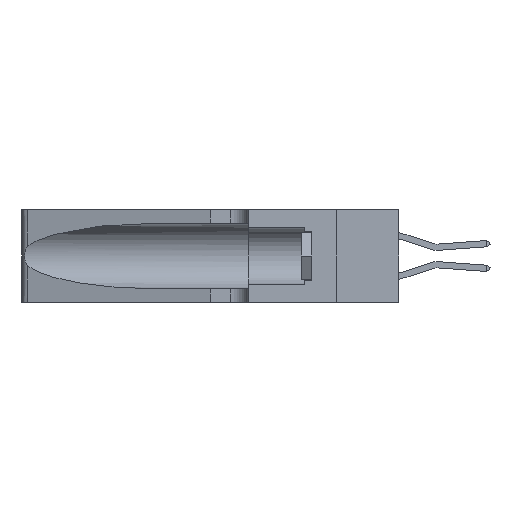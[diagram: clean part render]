
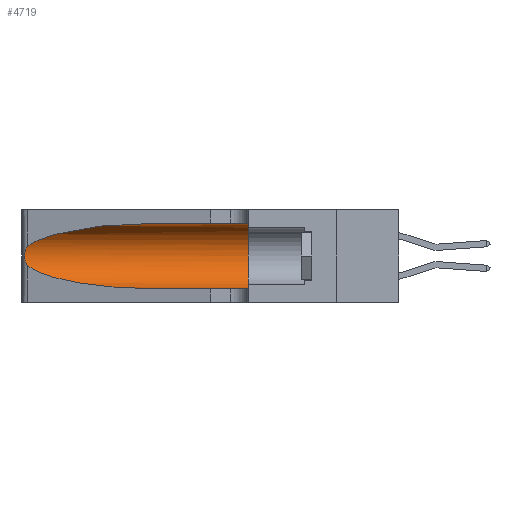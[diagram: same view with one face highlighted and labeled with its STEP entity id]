
A CAD part, left-side view. The second image highlights one B-rep face of the part: STEP entity #4719.
In plain terms, the highlighted cylindrical face has radius 3.308 mm (diameter 6.617 mm), a partial arc.
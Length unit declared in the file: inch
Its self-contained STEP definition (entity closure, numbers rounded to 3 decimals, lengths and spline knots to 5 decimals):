
#1466 = CARTESIAN_POINT ( 'NONE',  ( 0.18966, 0.96281, 0.05475 ) ) ;
#1653 = AXIS2_PLACEMENT_3D ( 'NONE', #7147, #27205, #10057 ) ;
#1807 = CARTESIAN_POINT ( 'NONE',  ( 0.25789, 1.23486, 0.15765 ) ) ;
#2402 = FACE_OUTER_BOUND ( 'NONE', #33620, .T. ) ;
#3666 = VERTEX_POINT ( 'NONE', #22885 ) ;
#3780 = EDGE_CURVE ( 'NONE', #10870, #3666, #19137, .T. ) ;
#3822 = CARTESIAN_POINT ( 'NONE',  ( 0.1305, 0.72297, 0.31525 ) ) ;
#4201 = CARTESIAN_POINT ( 'NONE',  ( 0.1305, 0.72297, 0.05475 ) ) ;
#4461 = DIRECTION ( 'NONE',  ( 0., -1., 0. ) ) ;
#4567 = CARTESIAN_POINT ( 'NONE',  ( 0.25487, 1.22718, 0.22369 ) ) ;
#4694 = CARTESIAN_POINT ( 'NONE',  ( 0.25555, 1.22993, 0.14849 ) ) ;
#4719 = ADVANCED_FACE ( 'NONE', ( #2402 ), #30220, .F. ) ;
#6784 = ORIENTED_EDGE ( 'NONE', *, *, #3780, .F. ) ;
#6940 =( BOUNDED_CURVE ( )  B_SPLINE_CURVE ( 3, ( #23970, #26809, #29705, #12562 ),
 .UNSPECIFIED., .F., .T. ) 
 B_SPLINE_CURVE_WITH_KNOTS ( ( 4, 4 ),
 ( 1.5708, 2.84003 ),
 .UNSPECIFIED. ) 
 CURVE ( )  GEOMETRIC_REPRESENTATION_ITEM ( )  RATIONAL_B_SPLINE_CURVE ( ( 1., 0.87, 0.87, 1. ) ) 
 REPRESENTATION_ITEM ( '' )  );
#7147 = CARTESIAN_POINT ( 'NONE',  ( 0.1305, 0.35, 0.185 ) ) ;
#7508 = CIRCLE ( 'NONE', #1653, 0.13025 ) ;
#7810 = DIRECTION ( 'NONE',  ( 0., -1., 0. ) ) ;
#8117 = ORIENTED_EDGE ( 'NONE', *, *, #17282, .T. ) ;
#9038 = VERTEX_POINT ( 'NONE', #9296 ) ;
#9296 = CARTESIAN_POINT ( 'NONE',  ( 0.25487, 1.22718, 0.22369 ) ) ;
#9963 = CARTESIAN_POINT ( 'NONE',  ( 0.1305, 0.35, 0.05475 ) ) ;
#10057 = DIRECTION ( 'NONE',  ( 0., 0., 1. ) ) ;
#10265 = DIRECTION ( 'NONE',  ( 0., 0., -1. ) ) ;
#10368 = CARTESIAN_POINT ( 'NONE',  ( 0.25787, 1.23484, 0.2124 ) ) ;
#10589 = VECTOR ( 'NONE', #20499, 39.37008 ) ;
#10870 = VERTEX_POINT ( 'NONE', #3822 ) ;
#11802 = AXIS2_PLACEMENT_3D ( 'NONE', #33036, #4461, #10265 ) ;
#12562 = CARTESIAN_POINT ( 'NONE',  ( 0.25487, 1.22718, 0.22369 ) ) ;
#12659 = ORIENTED_EDGE ( 'NONE', *, *, #28357, .F. ) ;
#13277 = CARTESIAN_POINT ( 'NONE',  ( 0.26018, 1.23835, 0.19895 ) ) ;
#13388 = CARTESIAN_POINT ( 'NONE',  ( 0.25487, 1.22718, 0.14631 ) ) ;
#13667 = B_SPLINE_CURVE_WITH_KNOTS ( 'NONE', 3,
 ( #4567, #21814, #27521, #10368, #30413, #13277, #33268, #16141, #36155, #19046, #1807, #21941, #4694, #24787 ),
 .UNSPECIFIED., .F., .F.,
 ( 4, 2, 2, 2, 2, 2, 4 ),
 ( 0., 0.00027, 0.00053, 0.00107, 0.0016, 0.00187, 0.00214 ),
 .UNSPECIFIED. ) ;
#15833 = CARTESIAN_POINT ( 'NONE',  ( 0.2373, 1.15595, 0.08982 ) ) ;
#16141 = CARTESIAN_POINT ( 'NONE',  ( 0.26075, 1.23896, 0.178 ) ) ;
#17192 = VERTEX_POINT ( 'NONE', #4201 ) ;
#17282 = EDGE_CURVE ( 'NONE', #9038, #24364, #13667, .T. ) ;
#17476 = VECTOR ( 'NONE', #7810, 39.37008 ) ;
#17594 = ORIENTED_EDGE ( 'NONE', *, *, #35436, .T. ) ;
#18437 = EDGE_CURVE ( 'NONE', #10870, #9038, #6940, .T. ) ;
#19046 = CARTESIAN_POINT ( 'NONE',  ( 0.25856, 1.23593, 0.16098 ) ) ;
#19137 = LINE ( 'NONE', #34708, #10589 ) ;
#20499 = DIRECTION ( 'NONE',  ( 0., -1., 0. ) ) ;
#21620 = CARTESIAN_POINT ( 'NONE',  ( 0.1305, 0.72297, 0.05475 ) ) ;
#21814 = CARTESIAN_POINT ( 'NONE',  ( 0.25555, 1.22994, 0.2215 ) ) ;
#21855 = EDGE_CURVE ( 'NONE', #17192, #29577, #24193, .T. ) ;
#21941 = CARTESIAN_POINT ( 'NONE',  ( 0.25639, 1.23186, 0.15144 ) ) ;
#22885 = CARTESIAN_POINT ( 'NONE',  ( 0.1305, 0.35, 0.31525 ) ) ;
#23970 = CARTESIAN_POINT ( 'NONE',  ( 0.1305, 0.72297, 0.31525 ) ) ;
#24193 = LINE ( 'NONE', #25008, #17476 ) ;
#24364 = VERTEX_POINT ( 'NONE', #13388 ) ;
#24787 = CARTESIAN_POINT ( 'NONE',  ( 0.25487, 1.22718, 0.14631 ) ) ;
#25008 = CARTESIAN_POINT ( 'NONE',  ( 0.1305, 1.61858, 0.05475 ) ) ;
#26809 = CARTESIAN_POINT ( 'NONE',  ( 0.18966, 0.96281, 0.31525 ) ) ;
#27205 = DIRECTION ( 'NONE',  ( 0., 1., 0. ) ) ;
#27521 = CARTESIAN_POINT ( 'NONE',  ( 0.25639, 1.23184, 0.21858 ) ) ;
#28357 = EDGE_CURVE ( 'NONE', #3666, #29577, #7508, .T. ) ;
#29577 = VERTEX_POINT ( 'NONE', #9963 ) ;
#29705 = CARTESIAN_POINT ( 'NONE',  ( 0.2373, 1.15595, 0.28018 ) ) ;
#30107 = ORIENTED_EDGE ( 'NONE', *, *, #18437, .T. ) ;
#30220 = CYLINDRICAL_SURFACE ( 'NONE', #11802, 0.13025 ) ;
#30413 = CARTESIAN_POINT ( 'NONE',  ( 0.25854, 1.2359, 0.20912 ) ) ;
#32781 = ORIENTED_EDGE ( 'NONE', *, *, #21855, .T. ) ;
#33036 = CARTESIAN_POINT ( 'NONE',  ( 0.1305, 1.61858, 0.185 ) ) ;
#33268 = CARTESIAN_POINT ( 'NONE',  ( 0.26075, 1.23896, 0.19203 ) ) ;
#33620 = EDGE_LOOP ( 'NONE', ( #30107, #8117, #17594, #32781, #12659, #6784 ) ) ;
#34708 = CARTESIAN_POINT ( 'NONE',  ( 0.1305, 1.61858, 0.31525 ) ) ;
#34711 =( BOUNDED_CURVE ( )  B_SPLINE_CURVE ( 3, ( #35817, #15833, #1466, #21620 ),
 .UNSPECIFIED., .F., .F. ) 
 B_SPLINE_CURVE_WITH_KNOTS ( ( 4, 4 ),
 ( 3.44316, 4.71239 ),
 .UNSPECIFIED. ) 
 CURVE ( )  GEOMETRIC_REPRESENTATION_ITEM ( )  RATIONAL_B_SPLINE_CURVE ( ( 1., 0.87, 0.87, 1. ) ) 
 REPRESENTATION_ITEM ( '' )  );
#35436 = EDGE_CURVE ( 'NONE', #24364, #17192, #34711, .T. ) ;
#35817 = CARTESIAN_POINT ( 'NONE',  ( 0.25487, 1.22718, 0.14631 ) ) ;
#36155 = CARTESIAN_POINT ( 'NONE',  ( 0.26017, 1.23833, 0.17102 ) ) ;
